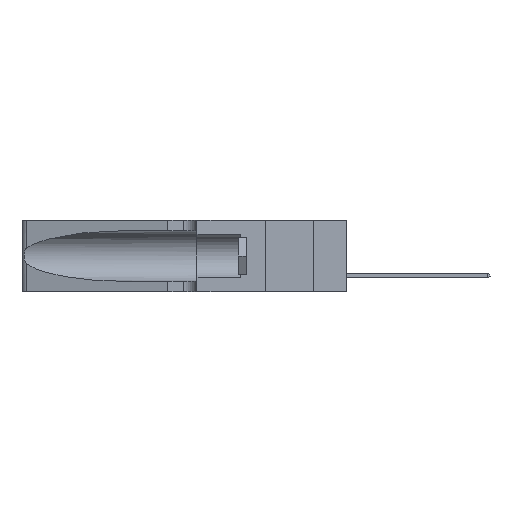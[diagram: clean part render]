
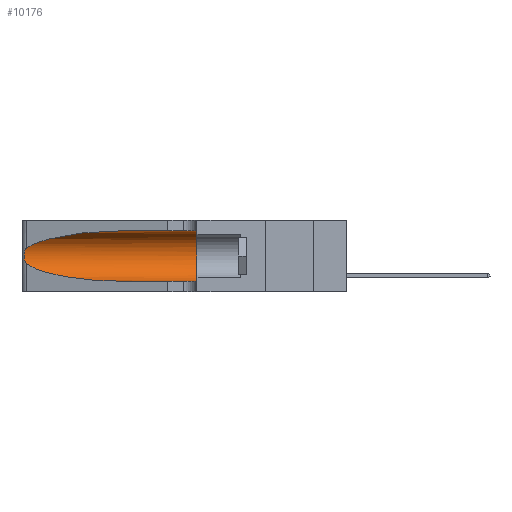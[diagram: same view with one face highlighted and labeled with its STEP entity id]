
A CAD part, left-side view. The second image highlights one B-rep face of the part: STEP entity #10176.
In plain terms, the highlighted cylindrical face has radius 3.308 mm (diameter 6.617 mm), a partial arc.
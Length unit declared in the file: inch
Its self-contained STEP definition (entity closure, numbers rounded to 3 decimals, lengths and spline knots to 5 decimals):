
#644 = EDGE_LOOP ( 'NONE', ( #29105, #24489, #14253, #3057, #7062, #19157 ) ) ;
#1392 = CARTESIAN_POINT ( 'NONE',  ( 0.26018, 1.23835, 0.19895 ) ) ;
#1843 = DIRECTION ( 'NONE',  ( 0., -1., 0. ) ) ;
#2562 = CARTESIAN_POINT ( 'NONE',  ( 0.25487, 1.22718, 0.22369 ) ) ;
#2859 = CARTESIAN_POINT ( 'NONE',  ( 0.2373, 1.15595, 0.08982 ) ) ;
#3057 = ORIENTED_EDGE ( 'NONE', *, *, #17872, .T. ) ;
#3060 = CYLINDRICAL_SURFACE ( 'NONE', #5257, 0.13025 ) ;
#3073 = CARTESIAN_POINT ( 'NONE',  ( 0.1305, 0.72297, 0.05475 ) ) ;
#4120 = CARTESIAN_POINT ( 'NONE',  ( 0.1305, 0.35, 0.05475 ) ) ;
#4596 = CARTESIAN_POINT ( 'NONE',  ( 0.26017, 1.23833, 0.17102 ) ) ;
#4923 = VECTOR ( 'NONE', #20055, 39.37008 ) ;
#5257 = AXIS2_PLACEMENT_3D ( 'NONE', #8136, #13106, #10377 ) ;
#6059 =( BOUNDED_CURVE ( )  B_SPLINE_CURVE ( 3, ( #24474, #2859, #29183, #3073 ),
 .UNSPECIFIED., .F., .T. ) 
 B_SPLINE_CURVE_WITH_KNOTS ( ( 4, 4 ),
 ( 3.44316, 4.71239 ),
 .UNSPECIFIED. ) 
 CURVE ( )  GEOMETRIC_REPRESENTATION_ITEM ( )  RATIONAL_B_SPLINE_CURVE ( ( 1., 0.87, 0.87, 1. ) ) 
 REPRESENTATION_ITEM ( '' )  );
#6456 = CARTESIAN_POINT ( 'NONE',  ( 0.25487, 1.22718, 0.22369 ) ) ;
#6753 = CARTESIAN_POINT ( 'NONE',  ( 0.25856, 1.23593, 0.16098 ) ) ;
#7062 = ORIENTED_EDGE ( 'NONE', *, *, #26666, .F. ) ;
#8136 = CARTESIAN_POINT ( 'NONE',  ( 0.1305, 1.61858, 0.185 ) ) ;
#8600 = CARTESIAN_POINT ( 'NONE',  ( 0.25639, 1.23184, 0.21858 ) ) ;
#8712 =( BOUNDED_CURVE ( )  B_SPLINE_CURVE ( 3, ( #26948, #17147, #10031, #24229 ),
 .UNSPECIFIED., .F., .F. ) 
 B_SPLINE_CURVE_WITH_KNOTS ( ( 4, 4 ),
 ( 1.5708, 2.84003 ),
 .UNSPECIFIED. ) 
 CURVE ( )  GEOMETRIC_REPRESENTATION_ITEM ( )  RATIONAL_B_SPLINE_CURVE ( ( 1., 0.87, 0.87, 1. ) ) 
 REPRESENTATION_ITEM ( '' )  );
#9024 = CARTESIAN_POINT ( 'NONE',  ( 0.25639, 1.23186, 0.15144 ) ) ;
#9192 = EDGE_CURVE ( 'NONE', #27769, #13855, #8712, .T. ) ;
#9414 = EDGE_CURVE ( 'NONE', #13855, #18150, #26842, .T. ) ;
#10031 = CARTESIAN_POINT ( 'NONE',  ( 0.2373, 1.15595, 0.28018 ) ) ;
#10176 = ADVANCED_FACE ( 'NONE', ( #29491 ), #3060, .F. ) ;
#10377 = DIRECTION ( 'NONE',  ( 0., 0., -1. ) ) ;
#10671 = EDGE_CURVE ( 'NONE', #27769, #15310, #29460, .T. ) ;
#10907 = CARTESIAN_POINT ( 'NONE',  ( 0.1305, 0.72297, 0.05475 ) ) ;
#11195 = CARTESIAN_POINT ( 'NONE',  ( 0.25854, 1.2359, 0.20912 ) ) ;
#11572 = LINE ( 'NONE', #12765, #4923 ) ;
#11736 = CARTESIAN_POINT ( 'NONE',  ( 0.1305, 1.61858, 0.31525 ) ) ;
#12355 = CARTESIAN_POINT ( 'NONE',  ( 0.1305, 0.35, 0.185 ) ) ;
#12376 = CIRCLE ( 'NONE', #27150, 0.13025 ) ;
#12765 = CARTESIAN_POINT ( 'NONE',  ( 0.1305, 1.61858, 0.05475 ) ) ;
#13106 = DIRECTION ( 'NONE',  ( 0., -1., 0. ) ) ;
#13855 = VERTEX_POINT ( 'NONE', #2562 ) ;
#14253 = ORIENTED_EDGE ( 'NONE', *, *, #28075, .T. ) ;
#14477 = VECTOR ( 'NONE', #1843, 39.37008 ) ;
#14854 = CARTESIAN_POINT ( 'NONE',  ( 0.25487, 1.22718, 0.14631 ) ) ;
#15310 = VERTEX_POINT ( 'NONE', #23592 ) ;
#15475 = CARTESIAN_POINT ( 'NONE',  ( 0.25787, 1.23484, 0.2124 ) ) ;
#16107 = CARTESIAN_POINT ( 'NONE',  ( 0.25487, 1.22718, 0.14631 ) ) ;
#17147 = CARTESIAN_POINT ( 'NONE',  ( 0.18966, 0.96281, 0.31525 ) ) ;
#17872 = EDGE_CURVE ( 'NONE', #30141, #21214, #11572, .T. ) ;
#17889 = CARTESIAN_POINT ( 'NONE',  ( 0.26075, 1.23896, 0.178 ) ) ;
#18150 = VERTEX_POINT ( 'NONE', #14854 ) ;
#19157 = ORIENTED_EDGE ( 'NONE', *, *, #10671, .F. ) ;
#20055 = DIRECTION ( 'NONE',  ( 0., -1., 0. ) ) ;
#21194 = CARTESIAN_POINT ( 'NONE',  ( 0.25555, 1.22993, 0.14849 ) ) ;
#21214 = VERTEX_POINT ( 'NONE', #4120 ) ;
#21535 = DIRECTION ( 'NONE',  ( 0., 1., 0. ) ) ;
#23105 = CARTESIAN_POINT ( 'NONE',  ( 0.25555, 1.22994, 0.2215 ) ) ;
#23592 = CARTESIAN_POINT ( 'NONE',  ( 0.1305, 0.35, 0.31525 ) ) ;
#24229 = CARTESIAN_POINT ( 'NONE',  ( 0.25487, 1.22718, 0.22369 ) ) ;
#24474 = CARTESIAN_POINT ( 'NONE',  ( 0.25487, 1.22718, 0.14631 ) ) ;
#24489 = ORIENTED_EDGE ( 'NONE', *, *, #9414, .T. ) ;
#25607 = CARTESIAN_POINT ( 'NONE',  ( 0.25789, 1.23486, 0.15765 ) ) ;
#25772 = CARTESIAN_POINT ( 'NONE',  ( 0.1305, 0.72297, 0.31525 ) ) ;
#26257 = DIRECTION ( 'NONE',  ( 0., 0., 1. ) ) ;
#26666 = EDGE_CURVE ( 'NONE', #15310, #21214, #12376, .T. ) ;
#26842 = B_SPLINE_CURVE_WITH_KNOTS ( 'NONE', 3,
 ( #6456, #23105, #8600, #15475, #11195, #1392, #27910, #17889, #4596, #6753, #25607, #9024, #21194, #16107 ),
 .UNSPECIFIED., .F., .F.,
 ( 4, 2, 2, 2, 2, 2, 4 ),
 ( 0., 0.00027, 0.00053, 0.00107, 0.0016, 0.00187, 0.00214 ),
 .UNSPECIFIED. ) ;
#26948 = CARTESIAN_POINT ( 'NONE',  ( 0.1305, 0.72297, 0.31525 ) ) ;
#27150 = AXIS2_PLACEMENT_3D ( 'NONE', #12355, #21535, #26257 ) ;
#27769 = VERTEX_POINT ( 'NONE', #25772 ) ;
#27910 = CARTESIAN_POINT ( 'NONE',  ( 0.26075, 1.23896, 0.19203 ) ) ;
#28075 = EDGE_CURVE ( 'NONE', #18150, #30141, #6059, .T. ) ;
#29105 = ORIENTED_EDGE ( 'NONE', *, *, #9192, .T. ) ;
#29183 = CARTESIAN_POINT ( 'NONE',  ( 0.18966, 0.96281, 0.05475 ) ) ;
#29460 = LINE ( 'NONE', #11736, #14477 ) ;
#29491 = FACE_OUTER_BOUND ( 'NONE', #644, .T. ) ;
#30141 = VERTEX_POINT ( 'NONE', #10907 ) ;
